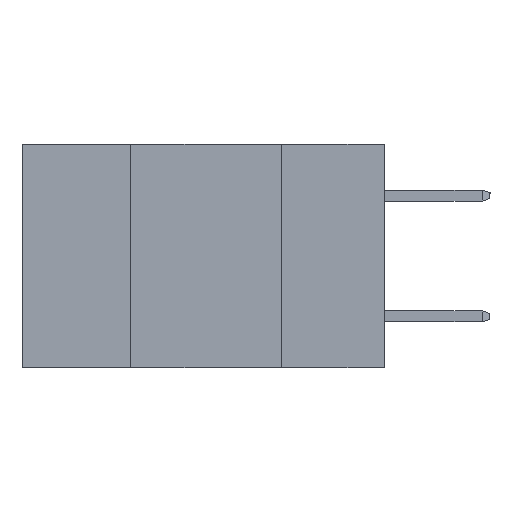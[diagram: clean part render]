
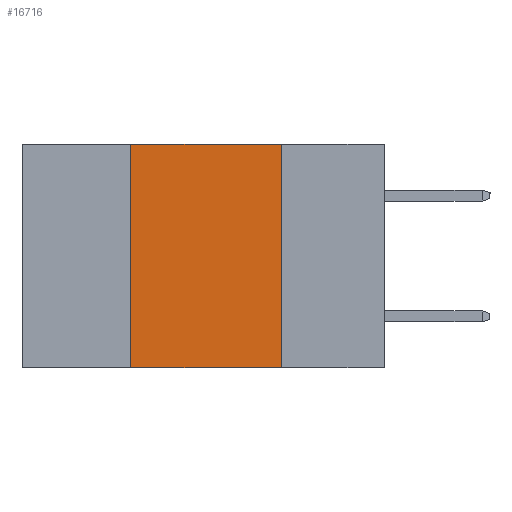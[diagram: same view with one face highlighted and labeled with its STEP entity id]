
A CAD part, left-side view. The second image highlights one B-rep face of the part: STEP entity #16716.
In plain terms, the highlighted planar face has unit normal (-1, 0, 0).
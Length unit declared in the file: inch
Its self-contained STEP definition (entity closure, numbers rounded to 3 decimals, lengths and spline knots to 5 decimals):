
#281 = DIRECTION ( 'NONE',  ( 1., 0., 0. ) ) ;
#417 = CARTESIAN_POINT ( 'NONE',  ( 0., 0.42, -0.37 ) ) ;
#500 = ORIENTED_EDGE ( 'NONE', *, *, #22419, .F. ) ;
#2604 = LINE ( 'NONE', #18469, #6934 ) ;
#3469 = DIRECTION ( 'NONE',  ( 0., 0., 1. ) ) ;
#4460 = VECTOR ( 'NONE', #3469, 39.37008 ) ;
#4790 = ORIENTED_EDGE ( 'NONE', *, *, #8730, .F. ) ;
#5667 = CARTESIAN_POINT ( 'NONE',  ( 0., 0.17, -0.37 ) ) ;
#6277 = CARTESIAN_POINT ( 'NONE',  ( 0., 0.6, 0. ) ) ;
#6934 = VECTOR ( 'NONE', #10147, 39.37008 ) ;
#6973 = CARTESIAN_POINT ( 'NONE',  ( 0., 0.42, -0.37 ) ) ;
#7233 = LINE ( 'NONE', #6973, #4460 ) ;
#7869 = EDGE_CURVE ( 'NONE', #9372, #12631, #10053, .T. ) ;
#8086 = VERTEX_POINT ( 'NONE', #22413 ) ;
#8730 = EDGE_CURVE ( 'NONE', #14835, #8086, #7233, .T. ) ;
#9372 = VERTEX_POINT ( 'NONE', #19265 ) ;
#10053 = LINE ( 'NONE', #5667, #15795 ) ;
#10147 = DIRECTION ( 'NONE',  ( 0., -1., 0. ) ) ;
#11927 = AXIS2_PLACEMENT_3D ( 'NONE', #6277, #281, #12375 ) ;
#11939 = LINE ( 'NONE', #24037, #16080 ) ;
#12375 = DIRECTION ( 'NONE',  ( 0., 0., -1. ) ) ;
#12631 = VERTEX_POINT ( 'NONE', #17416 ) ;
#13881 = DIRECTION ( 'NONE',  ( 0., -1., 0. ) ) ;
#14835 = VERTEX_POINT ( 'NONE', #417 ) ;
#15795 = VECTOR ( 'NONE', #16017, 39.37008 ) ;
#16017 = DIRECTION ( 'NONE',  ( 0., 0., -1. ) ) ;
#16080 = VECTOR ( 'NONE', #13881, 39.37008 ) ;
#16268 = PLANE ( 'NONE',  #11927 ) ;
#16533 = FACE_OUTER_BOUND ( 'NONE', #21755, .T. ) ;
#16716 = ADVANCED_FACE ( 'NONE', ( #16533 ), #16268, .F. ) ;
#17205 = ORIENTED_EDGE ( 'NONE', *, *, #7869, .F. ) ;
#17416 = CARTESIAN_POINT ( 'NONE',  ( 0., 0.17, -0.37 ) ) ;
#17955 = EDGE_CURVE ( 'NONE', #14835, #12631, #2604, .T. ) ;
#18469 = CARTESIAN_POINT ( 'NONE',  ( 0., 0.6, -0.37 ) ) ;
#19265 = CARTESIAN_POINT ( 'NONE',  ( 0., 0.17, 0. ) ) ;
#21755 = EDGE_LOOP ( 'NONE', ( #17205, #500, #4790, #22287 ) ) ;
#22287 = ORIENTED_EDGE ( 'NONE', *, *, #17955, .T. ) ;
#22413 = CARTESIAN_POINT ( 'NONE',  ( 0., 0.42, 0. ) ) ;
#22419 = EDGE_CURVE ( 'NONE', #8086, #9372, #11939, .T. ) ;
#24037 = CARTESIAN_POINT ( 'NONE',  ( 0., 0.6, 0. ) ) ;
